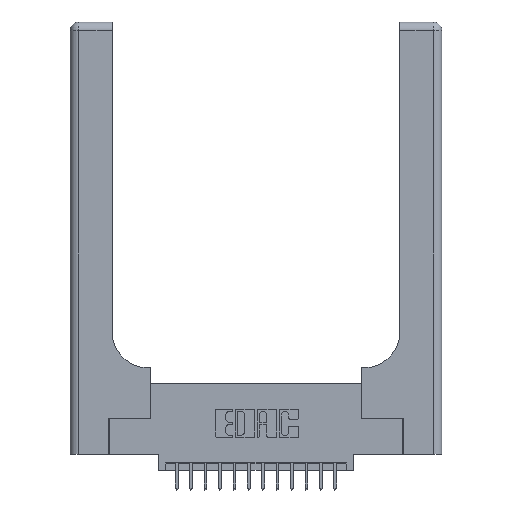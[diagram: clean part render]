
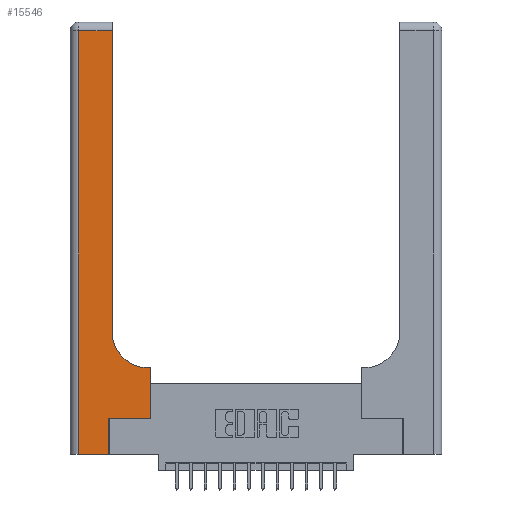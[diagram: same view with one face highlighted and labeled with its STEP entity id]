
A CAD part, top view. The second image highlights one B-rep face of the part: STEP entity #15546.
In plain terms, the highlighted planar face has unit normal (0, 0, 1).
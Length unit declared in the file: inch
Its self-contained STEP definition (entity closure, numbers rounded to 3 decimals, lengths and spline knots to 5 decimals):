
#23 = CARTESIAN_POINT ( 'NONE',  ( 0.06, 3., 0.37 ) ) ;
#129 = DIRECTION ( 'NONE',  ( 1., 0., 0. ) ) ;
#546 = DIRECTION ( 'NONE',  ( 0., 1., 0. ) ) ;
#596 = CARTESIAN_POINT ( 'NONE',  ( 0.5415, 0.6, 0.37 ) ) ;
#674 = AXIS2_PLACEMENT_3D ( 'NONE', #15121, #2133, #7974 ) ;
#1140 = FACE_OUTER_BOUND ( 'NONE', #14442, .T. ) ;
#1142 = EDGE_CURVE ( 'NONE', #9763, #5152, #2891, .T. ) ;
#1203 = DIRECTION ( 'NONE',  ( -1., 0., 0. ) ) ;
#1207 = DIRECTION ( 'NONE',  ( -1., 0., 0. ) ) ;
#1240 = EDGE_CURVE ( 'NONE', #5152, #12224, #1709, .T. ) ;
#1319 = DIRECTION ( 'NONE',  ( 0., 1., 0. ) ) ;
#1392 = EDGE_CURVE ( 'NONE', #4053, #2137, #9504, .T. ) ;
#1433 = LINE ( 'NONE', #23, #13495 ) ;
#1709 = LINE ( 'NONE', #5822, #11954 ) ;
#2133 = DIRECTION ( 'NONE',  ( 0., 0., -1. ) ) ;
#2137 = VERTEX_POINT ( 'NONE', #12741 ) ;
#2891 = LINE ( 'NONE', #10411, #17395 ) ;
#2929 = CARTESIAN_POINT ( 'NONE',  ( 0., 2.94, 0.37 ) ) ;
#3456 = ORIENTED_EDGE ( 'NONE', *, *, #1240, .T. ) ;
#4053 = VERTEX_POINT ( 'NONE', #596 ) ;
#4365 = LINE ( 'NONE', #2929, #12822 ) ;
#4434 = CARTESIAN_POINT ( 'NONE',  ( 0.06, 0., 0.37 ) ) ;
#4627 = AXIS2_PLACEMENT_3D ( 'NONE', #15256, #9740, #10996 ) ;
#5133 = ORIENTED_EDGE ( 'NONE', *, *, #14913, .T. ) ;
#5146 = PLANE ( 'NONE',  #4627 ) ;
#5152 = VERTEX_POINT ( 'NONE', #18336 ) ;
#5405 = VECTOR ( 'NONE', #1207, 39.37008 ) ;
#5579 = CARTESIAN_POINT ( 'NONE',  ( 0.2915, 2.94, 0.37 ) ) ;
#5822 = CARTESIAN_POINT ( 'NONE',  ( 0.269, 0.25, 0.37 ) ) ;
#6022 = DIRECTION ( 'NONE',  ( 0., 1., 0. ) ) ;
#6354 = EDGE_CURVE ( 'NONE', #12224, #18870, #14411, .T. ) ;
#6854 = CARTESIAN_POINT ( 'NONE',  ( 0.2915, 0.6, 0.37 ) ) ;
#7047 = VECTOR ( 'NONE', #17535, 39.37008 ) ;
#7974 = DIRECTION ( 'NONE',  ( 1., 0., 0. ) ) ;
#8169 = ORIENTED_EDGE ( 'NONE', *, *, #16230, .T. ) ;
#8795 = CARTESIAN_POINT ( 'NONE',  ( 0.06, 2.94, 0.37 ) ) ;
#9014 = CARTESIAN_POINT ( 'NONE',  ( 0.269, 0., 0.37 ) ) ;
#9028 = EDGE_CURVE ( 'NONE', #18870, #4053, #9990, .T. ) ;
#9074 = VECTOR ( 'NONE', #546, 39.37008 ) ;
#9153 = EDGE_CURVE ( 'NONE', #2137, #17738, #9313, .T. ) ;
#9313 = LINE ( 'NONE', #12115, #9074 ) ;
#9504 = CIRCLE ( 'NONE', #674, 0.25 ) ;
#9740 = DIRECTION ( 'NONE',  ( 0., 0., -1. ) ) ;
#9763 = VERTEX_POINT ( 'NONE', #9014 ) ;
#9990 = LINE ( 'NONE', #6854, #5405 ) ;
#10291 = CARTESIAN_POINT ( 'NONE',  ( 0.5585, 0.25, 0.37 ) ) ;
#10334 = ORIENTED_EDGE ( 'NONE', *, *, #1142, .T. ) ;
#10411 = CARTESIAN_POINT ( 'NONE',  ( 0.269, 0., 0.37 ) ) ;
#10996 = DIRECTION ( 'NONE',  ( -1., 0., 0. ) ) ;
#11736 = LINE ( 'NONE', #18787, #7047 ) ;
#11743 = EDGE_CURVE ( 'NONE', #17738, #12157, #4365, .T. ) ;
#11874 = DIRECTION ( 'NONE',  ( 0., -1., 0. ) ) ;
#11944 = VERTEX_POINT ( 'NONE', #4434 ) ;
#11954 = VECTOR ( 'NONE', #129, 39.37008 ) ;
#12115 = CARTESIAN_POINT ( 'NONE',  ( 0.2915, 3., 0.37 ) ) ;
#12157 = VERTEX_POINT ( 'NONE', #8795 ) ;
#12224 = VERTEX_POINT ( 'NONE', #16411 ) ;
#12741 = CARTESIAN_POINT ( 'NONE',  ( 0.2915, 0.85, 0.37 ) ) ;
#12822 = VECTOR ( 'NONE', #1203, 39.37008 ) ;
#13253 = ORIENTED_EDGE ( 'NONE', *, *, #9153, .T. ) ;
#13495 = VECTOR ( 'NONE', #11874, 39.37008 ) ;
#14411 = LINE ( 'NONE', #10291, #18468 ) ;
#14419 = ORIENTED_EDGE ( 'NONE', *, *, #9028, .T. ) ;
#14442 = EDGE_LOOP ( 'NONE', ( #13253, #16396, #8169, #5133, #10334, #3456, #16093, #14419, #17775 ) ) ;
#14913 = EDGE_CURVE ( 'NONE', #11944, #9763, #11736, .T. ) ;
#15121 = CARTESIAN_POINT ( 'NONE',  ( 0.5415, 0.85, 0.37 ) ) ;
#15256 = CARTESIAN_POINT ( 'NONE',  ( 0., 3., 0.37 ) ) ;
#15546 = ADVANCED_FACE ( 'NONE', ( #1140 ), #5146, .F. ) ;
#16093 = ORIENTED_EDGE ( 'NONE', *, *, #6354, .T. ) ;
#16139 = CARTESIAN_POINT ( 'NONE',  ( 0.5585, 0.6, 0.37 ) ) ;
#16230 = EDGE_CURVE ( 'NONE', #12157, #11944, #1433, .T. ) ;
#16396 = ORIENTED_EDGE ( 'NONE', *, *, #11743, .T. ) ;
#16411 = CARTESIAN_POINT ( 'NONE',  ( 0.5585, 0.25, 0.37 ) ) ;
#17395 = VECTOR ( 'NONE', #6022, 39.37008 ) ;
#17535 = DIRECTION ( 'NONE',  ( 1., 0., 0. ) ) ;
#17738 = VERTEX_POINT ( 'NONE', #5579 ) ;
#17775 = ORIENTED_EDGE ( 'NONE', *, *, #1392, .T. ) ;
#18336 = CARTESIAN_POINT ( 'NONE',  ( 0.269, 0.25, 0.37 ) ) ;
#18468 = VECTOR ( 'NONE', #1319, 39.37008 ) ;
#18787 = CARTESIAN_POINT ( 'NONE',  ( 0., 0., 0.37 ) ) ;
#18870 = VERTEX_POINT ( 'NONE', #16139 ) ;
